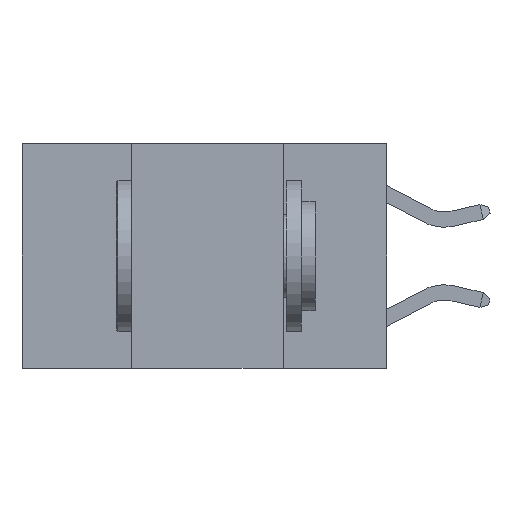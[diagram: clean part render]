
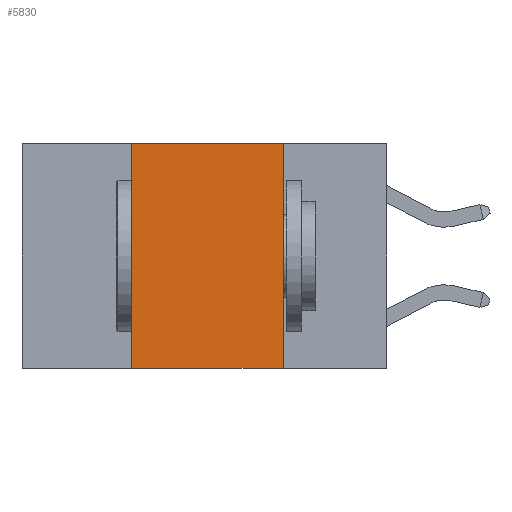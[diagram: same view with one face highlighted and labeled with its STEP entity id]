
A CAD part, left-side view. The second image highlights one B-rep face of the part: STEP entity #5830.
In plain terms, the highlighted planar face has unit normal (-1, 0, 0).
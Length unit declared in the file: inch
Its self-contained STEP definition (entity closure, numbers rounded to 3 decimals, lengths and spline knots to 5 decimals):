
#799 = ORIENTED_EDGE ( 'NONE', *, *, #16219, .F. ) ;
#1985 = VERTEX_POINT ( 'NONE', #11282 ) ;
#1986 = CARTESIAN_POINT ( 'NONE',  ( 0., 0.42, 0. ) ) ;
#2924 = VECTOR ( 'NONE', #13349, 39.37008 ) ;
#3938 = LINE ( 'NONE', #10063, #7346 ) ;
#4433 = CARTESIAN_POINT ( 'NONE',  ( 0., 0.17, 0. ) ) ;
#4499 = ORIENTED_EDGE ( 'NONE', *, *, #17169, .F. ) ;
#4745 = VERTEX_POINT ( 'NONE', #8421 ) ;
#4940 = ORIENTED_EDGE ( 'NONE', *, *, #14278, .T. ) ;
#5404 = AXIS2_PLACEMENT_3D ( 'NONE', #10764, #15183, #6429 ) ;
#5478 = LINE ( 'NONE', #16249, #2924 ) ;
#5830 = ADVANCED_FACE ( 'NONE', ( #8377 ), #15116, .F. ) ;
#6429 = DIRECTION ( 'NONE',  ( 0., 0., -1. ) ) ;
#7346 = VECTOR ( 'NONE', #11571, 39.37008 ) ;
#8321 = ORIENTED_EDGE ( 'NONE', *, *, #11959, .F. ) ;
#8377 = FACE_OUTER_BOUND ( 'NONE', #10484, .T. ) ;
#8421 = CARTESIAN_POINT ( 'NONE',  ( 0., 0.17, 0. ) ) ;
#9641 = DIRECTION ( 'NONE',  ( 0., 0., 1. ) ) ;
#10063 = CARTESIAN_POINT ( 'NONE',  ( 0., 0.6, 0. ) ) ;
#10484 = EDGE_LOOP ( 'NONE', ( #4499, #8321, #799, #4940 ) ) ;
#10764 = CARTESIAN_POINT ( 'NONE',  ( 0., 0.6, 0. ) ) ;
#10776 = CARTESIAN_POINT ( 'NONE',  ( 0., 0.42, -0.37 ) ) ;
#11282 = CARTESIAN_POINT ( 'NONE',  ( 0., 0.17, -0.37 ) ) ;
#11571 = DIRECTION ( 'NONE',  ( 0., -1., 0. ) ) ;
#11576 = VERTEX_POINT ( 'NONE', #10776 ) ;
#11959 = EDGE_CURVE ( 'NONE', #15097, #4745, #3938, .T. ) ;
#13166 = DIRECTION ( 'NONE',  ( 0., 0., -1. ) ) ;
#13349 = DIRECTION ( 'NONE',  ( 0., -1., 0. ) ) ;
#13597 = LINE ( 'NONE', #4433, #16977 ) ;
#14278 = EDGE_CURVE ( 'NONE', #11576, #1985, #5478, .T. ) ;
#14557 = VECTOR ( 'NONE', #9641, 39.37008 ) ;
#15097 = VERTEX_POINT ( 'NONE', #1986 ) ;
#15116 = PLANE ( 'NONE',  #5404 ) ;
#15183 = DIRECTION ( 'NONE',  ( 1., 0., 0. ) ) ;
#16219 = EDGE_CURVE ( 'NONE', #11576, #15097, #17910, .T. ) ;
#16249 = CARTESIAN_POINT ( 'NONE',  ( 0., 0.6, -0.37 ) ) ;
#16961 = CARTESIAN_POINT ( 'NONE',  ( 0., 0.42, 0. ) ) ;
#16977 = VECTOR ( 'NONE', #13166, 39.37008 ) ;
#17169 = EDGE_CURVE ( 'NONE', #4745, #1985, #13597, .T. ) ;
#17910 = LINE ( 'NONE', #16961, #14557 ) ;
